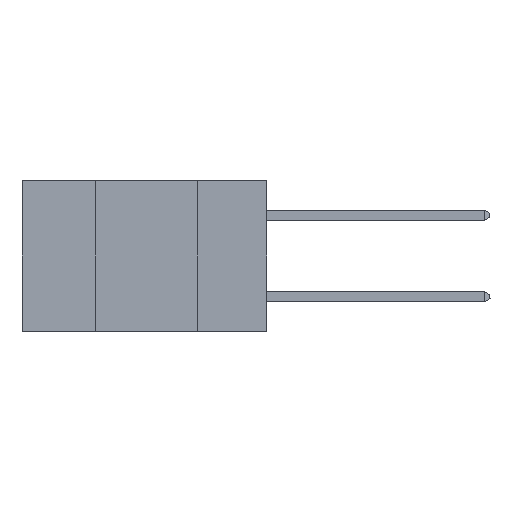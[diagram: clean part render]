
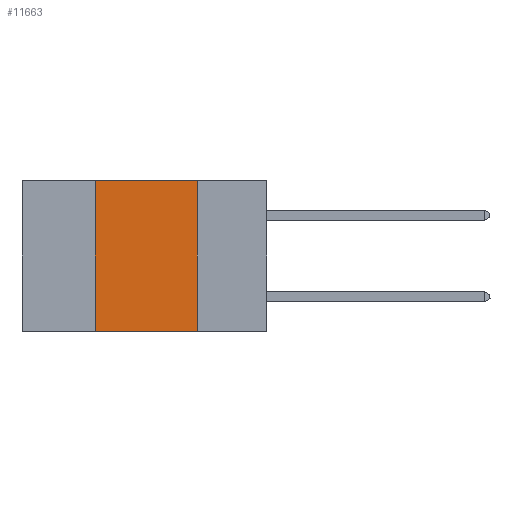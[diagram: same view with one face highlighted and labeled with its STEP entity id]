
A CAD part, left-side view. The second image highlights one B-rep face of the part: STEP entity #11663.
In plain terms, the highlighted planar face has unit normal (-1, 0, 0).
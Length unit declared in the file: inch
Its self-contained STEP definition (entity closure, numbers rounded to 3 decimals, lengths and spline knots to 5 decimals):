
#587 = VERTEX_POINT ( 'NONE', #15520 ) ;
#922 = ORIENTED_EDGE ( 'NONE', *, *, #18819, .T. ) ;
#1213 = ORIENTED_EDGE ( 'NONE', *, *, #12365, .F. ) ;
#2293 = DIRECTION ( 'NONE',  ( 0., 0., 1. ) ) ;
#3324 = VECTOR ( 'NONE', #19201, 39.37008 ) ;
#3959 = CARTESIAN_POINT ( 'NONE',  ( 0., 0.6, -0.37 ) ) ;
#5061 = PLANE ( 'NONE',  #6296 ) ;
#5914 = ORIENTED_EDGE ( 'NONE', *, *, #13662, .F. ) ;
#5925 = EDGE_LOOP ( 'NONE', ( #23614, #5914, #1213, #922 ) ) ;
#6296 = AXIS2_PLACEMENT_3D ( 'NONE', #12692, #10639, #23751 ) ;
#6636 = VECTOR ( 'NONE', #2293, 39.37008 ) ;
#6796 = VECTOR ( 'NONE', #23069, 39.37008 ) ;
#7716 = DIRECTION ( 'NONE',  ( 0., -1., 0. ) ) ;
#7871 = CARTESIAN_POINT ( 'NONE',  ( 0., 0.17, 0. ) ) ;
#8468 = FACE_OUTER_BOUND ( 'NONE', #5925, .T. ) ;
#9528 = CARTESIAN_POINT ( 'NONE',  ( 0., 0.6, 0. ) ) ;
#10065 = CARTESIAN_POINT ( 'NONE',  ( 0., 0.42, 0. ) ) ;
#10639 = DIRECTION ( 'NONE',  ( 1., 0., 0. ) ) ;
#11663 = ADVANCED_FACE ( 'NONE', ( #8468 ), #5061, .F. ) ;
#11937 = LINE ( 'NONE', #3959, #3324 ) ;
#11976 = VERTEX_POINT ( 'NONE', #12247 ) ;
#12247 = CARTESIAN_POINT ( 'NONE',  ( 0., 0.17, 0. ) ) ;
#12365 = EDGE_CURVE ( 'NONE', #20883, #587, #12879, .T. ) ;
#12692 = CARTESIAN_POINT ( 'NONE',  ( 0., 0.6, 0. ) ) ;
#12879 = LINE ( 'NONE', #10065, #6636 ) ;
#13662 = EDGE_CURVE ( 'NONE', #587, #11976, #22942, .T. ) ;
#13706 = CARTESIAN_POINT ( 'NONE',  ( 0., 0.42, -0.37 ) ) ;
#15520 = CARTESIAN_POINT ( 'NONE',  ( 0., 0.42, 0. ) ) ;
#16089 = LINE ( 'NONE', #7871, #6796 ) ;
#17906 = VECTOR ( 'NONE', #7716, 39.37008 ) ;
#18266 = CARTESIAN_POINT ( 'NONE',  ( 0., 0.17, -0.37 ) ) ;
#18819 = EDGE_CURVE ( 'NONE', #20883, #24636, #11937, .T. ) ;
#19191 = EDGE_CURVE ( 'NONE', #11976, #24636, #16089, .T. ) ;
#19201 = DIRECTION ( 'NONE',  ( 0., -1., 0. ) ) ;
#20883 = VERTEX_POINT ( 'NONE', #13706 ) ;
#22942 = LINE ( 'NONE', #9528, #17906 ) ;
#23069 = DIRECTION ( 'NONE',  ( 0., 0., -1. ) ) ;
#23614 = ORIENTED_EDGE ( 'NONE', *, *, #19191, .F. ) ;
#23751 = DIRECTION ( 'NONE',  ( 0., 0., -1. ) ) ;
#24636 = VERTEX_POINT ( 'NONE', #18266 ) ;
